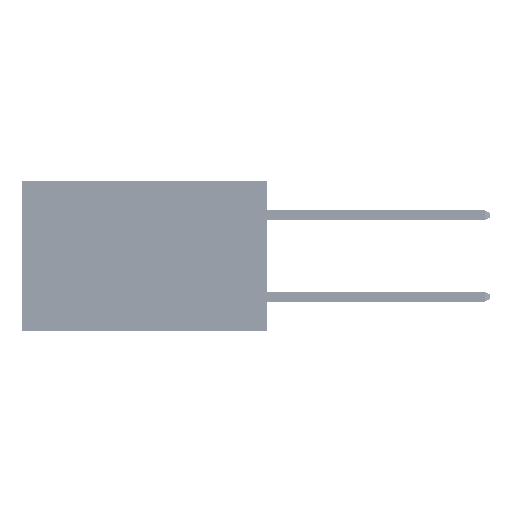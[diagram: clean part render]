
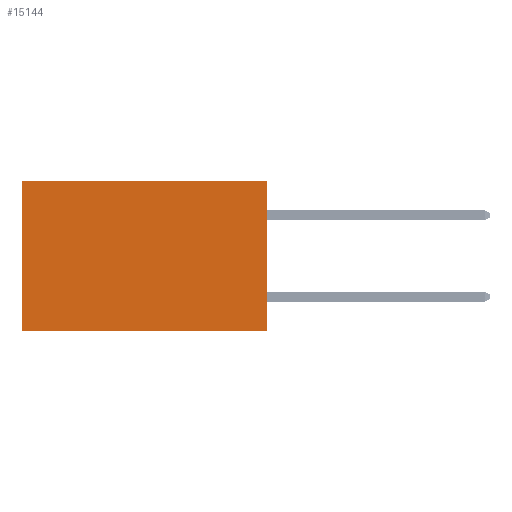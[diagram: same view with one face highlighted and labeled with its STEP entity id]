
A CAD part, left-side view. The second image highlights one B-rep face of the part: STEP entity #15144.
In plain terms, the highlighted planar face has unit normal (-1, 0, 0).
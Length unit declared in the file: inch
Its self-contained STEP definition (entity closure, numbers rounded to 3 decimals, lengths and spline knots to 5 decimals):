
#1434 = VECTOR ( 'NONE', #45025, 39.37008 ) ;
#3109 = VERTEX_POINT ( 'NONE', #15761 ) ;
#3350 = DIRECTION ( 'NONE',  ( 0., 0., -1. ) ) ;
#5316 = LINE ( 'NONE', #47605, #32494 ) ;
#9118 = CARTESIAN_POINT ( 'NONE',  ( 0.2875, 0., -0.37 ) ) ;
#9536 = CARTESIAN_POINT ( 'NONE',  ( 0.2875, 0., -0.37 ) ) ;
#9612 = VECTOR ( 'NONE', #16898, 39.37008 ) ;
#10799 = PLANE ( 'NONE',  #45261 ) ;
#11506 = LINE ( 'NONE', #41166, #1434 ) ;
#12291 = EDGE_CURVE ( 'NONE', #26591, #3109, #24803, .T. ) ;
#15144 = ADVANCED_FACE ( 'NONE', ( #16855 ), #10799, .F. ) ;
#15761 = CARTESIAN_POINT ( 'NONE',  ( 0.2875, 0.6, -0.37 ) ) ;
#16855 = FACE_OUTER_BOUND ( 'NONE', #27688, .T. ) ;
#16898 = DIRECTION ( 'NONE',  ( 0., 0., -1. ) ) ;
#19084 = VERTEX_POINT ( 'NONE', #44980 ) ;
#20983 = DIRECTION ( 'NONE',  ( 0., 1., 0. ) ) ;
#23724 = EDGE_CURVE ( 'NONE', #19084, #35357, #11506, .T. ) ;
#24803 = LINE ( 'NONE', #9536, #36557 ) ;
#26591 = VERTEX_POINT ( 'NONE', #9118 ) ;
#27513 = ORIENTED_EDGE ( 'NONE', *, *, #12291, .F. ) ;
#27622 = ORIENTED_EDGE ( 'NONE', *, *, #23724, .T. ) ;
#27688 = EDGE_LOOP ( 'NONE', ( #42279, #27513, #28792, #27622 ) ) ;
#28792 = ORIENTED_EDGE ( 'NONE', *, *, #41494, .F. ) ;
#32494 = VECTOR ( 'NONE', #40448, 39.37008 ) ;
#33548 = CARTESIAN_POINT ( 'NONE',  ( 0.2875, 0., 0. ) ) ;
#35357 = VERTEX_POINT ( 'NONE', #40752 ) ;
#36557 = VECTOR ( 'NONE', #20983, 39.37008 ) ;
#37030 = DIRECTION ( 'NONE',  ( 1., 0., 0. ) ) ;
#40448 = DIRECTION ( 'NONE',  ( 0., 0., -1. ) ) ;
#40752 = CARTESIAN_POINT ( 'NONE',  ( 0.2875, 0.6, 0. ) ) ;
#41166 = CARTESIAN_POINT ( 'NONE',  ( 0.2875, 0., 0. ) ) ;
#41494 = EDGE_CURVE ( 'NONE', #19084, #26591, #5316, .T. ) ;
#41564 = LINE ( 'NONE', #47753, #9612 ) ;
#42279 = ORIENTED_EDGE ( 'NONE', *, *, #47972, .T. ) ;
#44980 = CARTESIAN_POINT ( 'NONE',  ( 0.2875, 0., 0. ) ) ;
#45025 = DIRECTION ( 'NONE',  ( 0., 1., 0. ) ) ;
#45261 = AXIS2_PLACEMENT_3D ( 'NONE', #33548, #37030, #3350 ) ;
#47605 = CARTESIAN_POINT ( 'NONE',  ( 0.2875, 0., 0. ) ) ;
#47753 = CARTESIAN_POINT ( 'NONE',  ( 0.2875, 0.6, 0. ) ) ;
#47972 = EDGE_CURVE ( 'NONE', #35357, #3109, #41564, .T. ) ;
